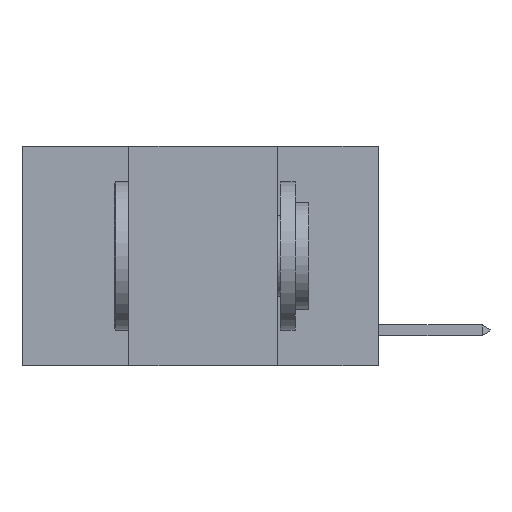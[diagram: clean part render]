
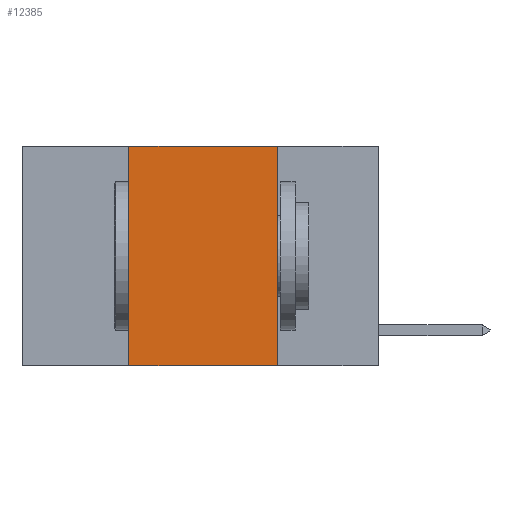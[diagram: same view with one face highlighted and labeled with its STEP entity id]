
A CAD part, left-side view. The second image highlights one B-rep face of the part: STEP entity #12385.
In plain terms, the highlighted planar face has unit normal (-1, 0, 0).
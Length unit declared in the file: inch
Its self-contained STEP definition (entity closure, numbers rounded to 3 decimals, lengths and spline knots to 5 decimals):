
#78 = VECTOR ( 'NONE', #3433, 39.37008 ) ;
#1701 = EDGE_LOOP ( 'NONE', ( #4348, #5492, #12615, #5763 ) ) ;
#2357 = AXIS2_PLACEMENT_3D ( 'NONE', #7930, #7972, #10852 ) ;
#3186 = CARTESIAN_POINT ( 'NONE',  ( 0., 0.17, -0.37 ) ) ;
#3433 = DIRECTION ( 'NONE',  ( 0., 0., 1. ) ) ;
#4072 = EDGE_CURVE ( 'NONE', #11409, #9333, #10509, .T. ) ;
#4348 = ORIENTED_EDGE ( 'NONE', *, *, #4072, .F. ) ;
#4957 = DIRECTION ( 'NONE',  ( 0., -1., 0. ) ) ;
#5492 = ORIENTED_EDGE ( 'NONE', *, *, #11105, .F. ) ;
#5763 = ORIENTED_EDGE ( 'NONE', *, *, #10673, .T. ) ;
#5868 = VECTOR ( 'NONE', #11295, 39.37008 ) ;
#5883 = LINE ( 'NONE', #6175, #78 ) ;
#6175 = CARTESIAN_POINT ( 'NONE',  ( 0., 0.42, 0. ) ) ;
#6190 = EDGE_CURVE ( 'NONE', #7992, #11853, #5883, .T. ) ;
#7389 = DIRECTION ( 'NONE',  ( 0., -1., 0. ) ) ;
#7774 = LINE ( 'NONE', #10988, #9022 ) ;
#7930 = CARTESIAN_POINT ( 'NONE',  ( 0., 0.6, 0. ) ) ;
#7947 = CARTESIAN_POINT ( 'NONE',  ( 0., 0.42, -0.37 ) ) ;
#7972 = DIRECTION ( 'NONE',  ( 1., 0., 0. ) ) ;
#7992 = VERTEX_POINT ( 'NONE', #7947 ) ;
#8323 = CARTESIAN_POINT ( 'NONE',  ( 0., 0.17, 0. ) ) ;
#8771 = CARTESIAN_POINT ( 'NONE',  ( 0., 0.6, -0.37 ) ) ;
#9022 = VECTOR ( 'NONE', #7389, 39.37008 ) ;
#9298 = LINE ( 'NONE', #8771, #12269 ) ;
#9333 = VERTEX_POINT ( 'NONE', #3186 ) ;
#9840 = PLANE ( 'NONE',  #2357 ) ;
#9938 = CARTESIAN_POINT ( 'NONE',  ( 0., 0.42, 0. ) ) ;
#10509 = LINE ( 'NONE', #8323, #5868 ) ;
#10673 = EDGE_CURVE ( 'NONE', #7992, #9333, #9298, .T. ) ;
#10852 = DIRECTION ( 'NONE',  ( 0., 0., -1. ) ) ;
#10988 = CARTESIAN_POINT ( 'NONE',  ( 0., 0.6, 0. ) ) ;
#11105 = EDGE_CURVE ( 'NONE', #11853, #11409, #7774, .T. ) ;
#11199 = CARTESIAN_POINT ( 'NONE',  ( 0., 0.17, 0. ) ) ;
#11295 = DIRECTION ( 'NONE',  ( 0., 0., -1. ) ) ;
#11409 = VERTEX_POINT ( 'NONE', #11199 ) ;
#11853 = VERTEX_POINT ( 'NONE', #9938 ) ;
#12269 = VECTOR ( 'NONE', #4957, 39.37008 ) ;
#12385 = ADVANCED_FACE ( 'NONE', ( #12853 ), #9840, .F. ) ;
#12615 = ORIENTED_EDGE ( 'NONE', *, *, #6190, .F. ) ;
#12853 = FACE_OUTER_BOUND ( 'NONE', #1701, .T. ) ;
